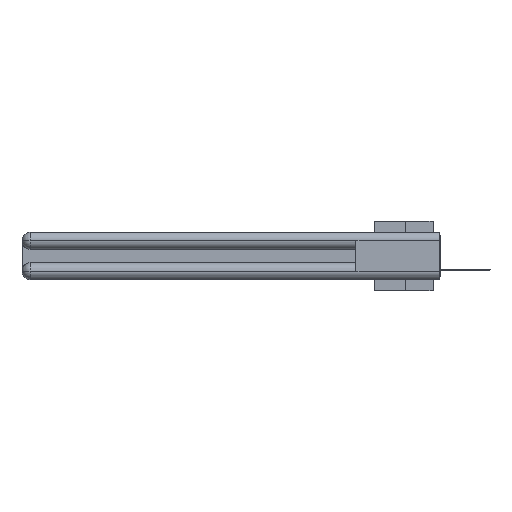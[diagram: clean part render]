
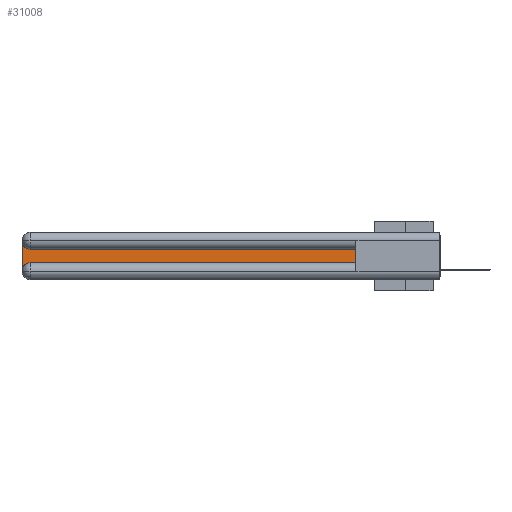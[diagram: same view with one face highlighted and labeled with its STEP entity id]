
A CAD part, left-side view. The second image highlights one B-rep face of the part: STEP entity #31008.
In plain terms, the highlighted planar face has unit normal (-1, 0, 0).
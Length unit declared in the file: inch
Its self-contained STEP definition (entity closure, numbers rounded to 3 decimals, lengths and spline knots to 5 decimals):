
#1441 = CARTESIAN_POINT ( 'NONE',  ( 0.075, 0.6, -0.1225 ) ) ;
#4202 = EDGE_CURVE ( 'NONE', #17600, #14054, #26633, .T. ) ;
#4354 = ORIENTED_EDGE ( 'NONE', *, *, #18242, .T. ) ;
#5284 = ORIENTED_EDGE ( 'NONE', *, *, #22229, .T. ) ;
#9069 = VERTEX_POINT ( 'NONE', #29560 ) ;
#9912 = CARTESIAN_POINT ( 'NONE',  ( 0.075, 3., -0.1225 ) ) ;
#10116 = CARTESIAN_POINT ( 'NONE',  ( 0.075, 0.6, -0.1225 ) ) ;
#10268 = VECTOR ( 'NONE', #10423, 39.37008 ) ;
#10423 = DIRECTION ( 'NONE',  ( 0., 0., -1. ) ) ;
#11735 = CARTESIAN_POINT ( 'NONE',  ( 0.075, 0.6, -0.2175 ) ) ;
#12723 = CARTESIAN_POINT ( 'NONE',  ( 0.075, 3., -0.2775 ) ) ;
#12823 = CARTESIAN_POINT ( 'NONE',  ( 0.075, 2.94, -0.0625 ) ) ;
#14054 = VERTEX_POINT ( 'NONE', #10116 ) ;
#14149 = ORIENTED_EDGE ( 'NONE', *, *, #22178, .T. ) ;
#14394 = AXIS2_PLACEMENT_3D ( 'NONE', #12823, #18384, #30059 ) ;
#14574 = EDGE_CURVE ( 'NONE', #14054, #29403, #15805, .T. ) ;
#15586 = DIRECTION ( 'NONE',  ( 0., 0., -1. ) ) ;
#15805 = LINE ( 'NONE', #1441, #17242 ) ;
#16157 = LINE ( 'NONE', #36662, #10268 ) ;
#16260 = AXIS2_PLACEMENT_3D ( 'NONE', #18824, #24200, #15586 ) ;
#17242 = VECTOR ( 'NONE', #36313, 39.37008 ) ;
#17600 = VERTEX_POINT ( 'NONE', #24210 ) ;
#18078 = EDGE_LOOP ( 'NONE', ( #29097, #5284, #18876, #4354, #14149, #21125 ) ) ;
#18242 = EDGE_CURVE ( 'NONE', #21207, #32838, #27434, .T. ) ;
#18384 = DIRECTION ( 'NONE',  ( 1., 0., 0. ) ) ;
#18664 = CARTESIAN_POINT ( 'NONE',  ( 0.075, 2.94, -0.2175 ) ) ;
#18824 = CARTESIAN_POINT ( 'NONE',  ( 0.075, 2.94, -0.2775 ) ) ;
#18876 = ORIENTED_EDGE ( 'NONE', *, *, #21324, .T. ) ;
#19456 = FACE_OUTER_BOUND ( 'NONE', #18078, .T. ) ;
#20584 = AXIS2_PLACEMENT_3D ( 'NONE', #9912, #21585, #22140 ) ;
#21125 = ORIENTED_EDGE ( 'NONE', *, *, #4202, .T. ) ;
#21207 = VERTEX_POINT ( 'NONE', #12723 ) ;
#21324 = EDGE_CURVE ( 'NONE', #9069, #21207, #16157, .T. ) ;
#21585 = DIRECTION ( 'NONE',  ( 1., 0., 0. ) ) ;
#22140 = DIRECTION ( 'NONE',  ( 0., 0., -1. ) ) ;
#22178 = EDGE_CURVE ( 'NONE', #32838, #17600, #30435, .T. ) ;
#22229 = EDGE_CURVE ( 'NONE', #29403, #9069, #27230, .T. ) ;
#23588 = DIRECTION ( 'NONE',  ( 0., 0., 1. ) ) ;
#24200 = DIRECTION ( 'NONE',  ( 1., 0., 0. ) ) ;
#24210 = CARTESIAN_POINT ( 'NONE',  ( 0.075, 0.6, -0.2175 ) ) ;
#24305 = CARTESIAN_POINT ( 'NONE',  ( 0.075, 0.6, -0.2175 ) ) ;
#26336 = CARTESIAN_POINT ( 'NONE',  ( 0.075, 2.94, -0.1225 ) ) ;
#26633 = LINE ( 'NONE', #11735, #31919 ) ;
#27181 = DIRECTION ( 'NONE',  ( 0., -1., 0. ) ) ;
#27230 = CIRCLE ( 'NONE', #14394, 0.06 ) ;
#27434 = CIRCLE ( 'NONE', #16260, 0.06 ) ;
#28059 = PLANE ( 'NONE',  #20584 ) ;
#29097 = ORIENTED_EDGE ( 'NONE', *, *, #14574, .T. ) ;
#29403 = VERTEX_POINT ( 'NONE', #26336 ) ;
#29560 = CARTESIAN_POINT ( 'NONE',  ( 0.075, 3., -0.0625 ) ) ;
#30059 = DIRECTION ( 'NONE',  ( 0., 0., -1. ) ) ;
#30435 = LINE ( 'NONE', #24305, #35168 ) ;
#31008 = ADVANCED_FACE ( 'NONE', ( #19456 ), #28059, .F. ) ;
#31919 = VECTOR ( 'NONE', #23588, 39.37008 ) ;
#32838 = VERTEX_POINT ( 'NONE', #18664 ) ;
#35168 = VECTOR ( 'NONE', #27181, 39.37008 ) ;
#36313 = DIRECTION ( 'NONE',  ( 0., 1., 0. ) ) ;
#36662 = CARTESIAN_POINT ( 'NONE',  ( 0.075, 3., -0.2175 ) ) ;
